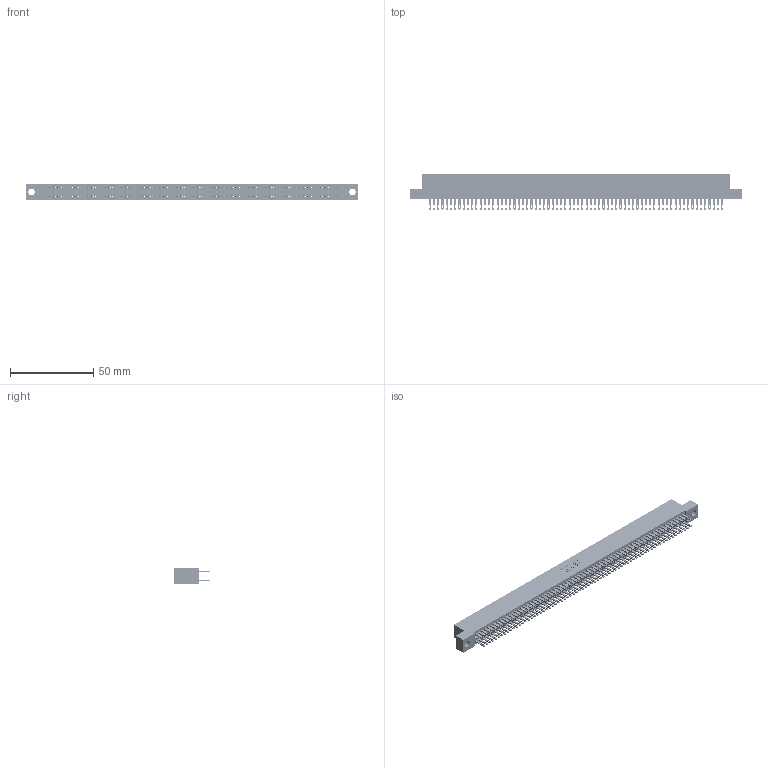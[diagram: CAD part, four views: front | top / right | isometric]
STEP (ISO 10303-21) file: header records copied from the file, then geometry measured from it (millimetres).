
FILE_DESCRIPTION (( 'STEP AP203' ), '1' );
FILE_NAME ('895-140-500-204.STEP', '2020-10-13T19:18:09', ( '' ), ( '' ), 'SwSTEP 2.0', 'SolidWorks 2020', '' );
FILE_SCHEMA (( 'CONFIG_CONTROL_DESIGN' ));
Length unit declared in the file: inch
Products named in the file (3): 345-292-001_345-293-100; 895-140-500-204; 845 Part_Flush Mounting Lugs - 0.156 Dia-TH
Assembly tree (141 placements, depth 2):
  895-140-500-204
    845 Part_Flush Mounting Lugs - 0.156 Dia-TH
    345-292-001_345-293-100  x140
Bounding box: 199.01 x 21.51 x 9.4 mm (x, y, z)
Volume: 19931.8 mm3; surface area: 31247.9 mm2
Topology: 141 solids, 141 shells, 6566 faces, 20081 edges, 13386 vertices
Faces by surface type: plane 3860, cylinder 2706
Entity records: 51087 total; most frequent: CARTESIAN_POINT 8536, ORIENTED_EDGE 8470, DIRECTION 7495, EDGE_CURVE 4235, LINE 3819, VECTOR 3819, VERTEX_POINT 2822, AXIS2_PLACEMENT_3D 1838
